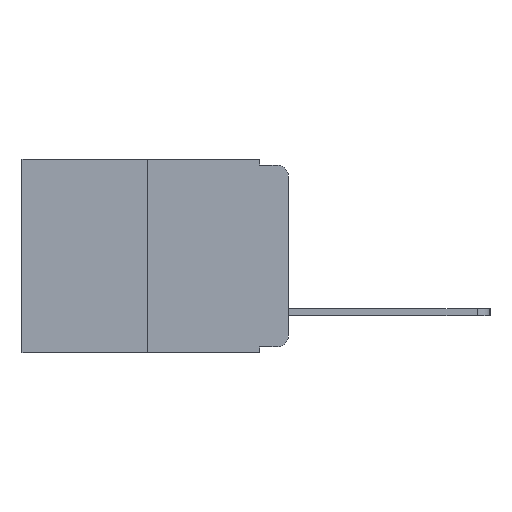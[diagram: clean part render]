
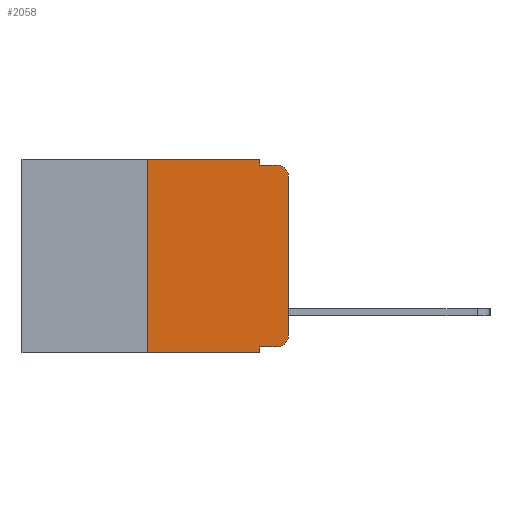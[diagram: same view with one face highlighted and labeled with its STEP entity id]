
A CAD part, left-side view. The second image highlights one B-rep face of the part: STEP entity #2058.
In plain terms, the highlighted planar face has unit normal (-1, 0, 0).
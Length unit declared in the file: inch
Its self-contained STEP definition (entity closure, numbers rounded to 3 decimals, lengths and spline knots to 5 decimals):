
#37 = CARTESIAN_POINT ( 'NONE',  ( 0., 0.473, 0. ) ) ;
#386 = VERTEX_POINT ( 'NONE', #9919 ) ;
#530 = CARTESIAN_POINT ( 'NONE',  ( 0., 0.051, -0.01 ) ) ;
#548 = CARTESIAN_POINT ( 'NONE',  ( 0., 0.25, -0.343 ) ) ;
#613 = CARTESIAN_POINT ( 'NONE',  ( 0., 0.25, 0. ) ) ;
#622 = CARTESIAN_POINT ( 'NONE',  ( 0., 0.051, -0.343 ) ) ;
#723 = VERTEX_POINT ( 'NONE', #8777 ) ;
#770 = EDGE_CURVE ( 'NONE', #386, #3956, #5890, .T. ) ;
#840 = CARTESIAN_POINT ( 'NONE',  ( 0., 0.051, 0. ) ) ;
#982 = AXIS2_PLACEMENT_3D ( 'NONE', #9594, #1736, #2177 ) ;
#1002 = EDGE_CURVE ( 'NONE', #3956, #3250, #6279, .T. ) ;
#1296 = VERTEX_POINT ( 'NONE', #622 ) ;
#1476 = VECTOR ( 'NONE', #10918, 39.37008 ) ;
#1736 = DIRECTION ( 'NONE',  ( -1., 0., 0. ) ) ;
#1944 = CARTESIAN_POINT ( 'NONE',  ( 0., 0.473, -0.343 ) ) ;
#2058 = ADVANCED_FACE ( 'NONE', ( #9789 ), #3217, .F. ) ;
#2126 = CARTESIAN_POINT ( 'NONE',  ( 0., 0.02, -0.03 ) ) ;
#2177 = DIRECTION ( 'NONE',  ( 0., 0., -1. ) ) ;
#2470 = DIRECTION ( 'NONE',  ( 0., 0., -1. ) ) ;
#2639 = CARTESIAN_POINT ( 'NONE',  ( 0., 0.051, 0. ) ) ;
#2712 = CIRCLE ( 'NONE', #9342, 0.02 ) ;
#2959 = DIRECTION ( 'NONE',  ( 0., -1., 0. ) ) ;
#3016 = ORIENTED_EDGE ( 'NONE', *, *, #10028, .T. ) ;
#3132 = DIRECTION ( 'NONE',  ( 0., 0., -1. ) ) ;
#3217 = PLANE ( 'NONE',  #4641 ) ;
#3250 = VERTEX_POINT ( 'NONE', #7295 ) ;
#3432 = VECTOR ( 'NONE', #5624, 39.37008 ) ;
#3616 = ORIENTED_EDGE ( 'NONE', *, *, #11093, .T. ) ;
#3637 = EDGE_CURVE ( 'NONE', #5778, #6204, #8328, .T. ) ;
#3664 = EDGE_CURVE ( 'NONE', #8264, #386, #10797, .T. ) ;
#3861 = VECTOR ( 'NONE', #7479, 39.37008 ) ;
#3956 = VERTEX_POINT ( 'NONE', #840 ) ;
#4050 = EDGE_LOOP ( 'NONE', ( #3016, #3616, #4286, #4614, #4967, #5254, #5357, #5860, #6402, #6733 ) ) ;
#4079 = LINE ( 'NONE', #2639, #1476 ) ;
#4286 = ORIENTED_EDGE ( 'NONE', *, *, #6363, .F. ) ;
#4368 = CARTESIAN_POINT ( 'NONE',  ( 0., 0.051, -0.333 ) ) ;
#4608 = CARTESIAN_POINT ( 'NONE',  ( 0., 0.02, -0.333 ) ) ;
#4614 = ORIENTED_EDGE ( 'NONE', *, *, #1002, .F. ) ;
#4641 = AXIS2_PLACEMENT_3D ( 'NONE', #37, #7239, #2470 ) ;
#4967 = ORIENTED_EDGE ( 'NONE', *, *, #770, .F. ) ;
#5078 = LINE ( 'NONE', #530, #9950 ) ;
#5254 = ORIENTED_EDGE ( 'NONE', *, *, #3664, .F. ) ;
#5357 = ORIENTED_EDGE ( 'NONE', *, *, #7666, .T. ) ;
#5373 = VECTOR ( 'NONE', #10734, 39.37008 ) ;
#5415 = EDGE_CURVE ( 'NONE', #9108, #1296, #4079, .T. ) ;
#5531 = DIRECTION ( 'NONE',  ( 0., -1., 0. ) ) ;
#5624 = DIRECTION ( 'NONE',  ( 0., -1., 0. ) ) ;
#5778 = VERTEX_POINT ( 'NONE', #4608 ) ;
#5860 = ORIENTED_EDGE ( 'NONE', *, *, #5415, .F. ) ;
#5890 = LINE ( 'NONE', #6013, #3432 ) ;
#6013 = CARTESIAN_POINT ( 'NONE',  ( 0., 0.473, 0. ) ) ;
#6204 = VERTEX_POINT ( 'NONE', #8804 ) ;
#6270 = VECTOR ( 'NONE', #6293, 39.37008 ) ;
#6279 = LINE ( 'NONE', #9103, #3861 ) ;
#6293 = DIRECTION ( 'NONE',  ( 0., 0., 1. ) ) ;
#6330 = CARTESIAN_POINT ( 'NONE',  ( 0., 0.02, -0.01 ) ) ;
#6363 = EDGE_CURVE ( 'NONE', #3250, #8302, #5078, .T. ) ;
#6402 = ORIENTED_EDGE ( 'NONE', *, *, #11432, .T. ) ;
#6509 = CARTESIAN_POINT ( 'NONE',  ( 0., 0., 0. ) ) ;
#6733 = ORIENTED_EDGE ( 'NONE', *, *, #3637, .T. ) ;
#7239 = DIRECTION ( 'NONE',  ( 1., 0., 0. ) ) ;
#7295 = CARTESIAN_POINT ( 'NONE',  ( 0., 0.051, -0.01 ) ) ;
#7479 = DIRECTION ( 'NONE',  ( 0., 0., -1. ) ) ;
#7666 = EDGE_CURVE ( 'NONE', #8264, #1296, #9923, .T. ) ;
#7689 = VECTOR ( 'NONE', #2959, 39.37008 ) ;
#8053 = DIRECTION ( 'NONE',  ( 0., -1., 0. ) ) ;
#8143 = CARTESIAN_POINT ( 'NONE',  ( 0., 0.051, -0.333 ) ) ;
#8264 = VERTEX_POINT ( 'NONE', #548 ) ;
#8302 = VERTEX_POINT ( 'NONE', #6330 ) ;
#8328 = CIRCLE ( 'NONE', #982, 0.02 ) ;
#8523 = DIRECTION ( 'NONE',  ( -1., 0., 0. ) ) ;
#8777 = CARTESIAN_POINT ( 'NONE',  ( 0., 0., -0.03 ) ) ;
#8804 = CARTESIAN_POINT ( 'NONE',  ( 0., 0., -0.313 ) ) ;
#9103 = CARTESIAN_POINT ( 'NONE',  ( 0., 0.051, 0. ) ) ;
#9108 = VERTEX_POINT ( 'NONE', #4368 ) ;
#9167 = VECTOR ( 'NONE', #5531, 39.37008 ) ;
#9342 = AXIS2_PLACEMENT_3D ( 'NONE', #2126, #8523, #3132 ) ;
#9594 = CARTESIAN_POINT ( 'NONE',  ( 0., 0.02, -0.313 ) ) ;
#9789 = FACE_OUTER_BOUND ( 'NONE', #4050, .T. ) ;
#9919 = CARTESIAN_POINT ( 'NONE',  ( 0., 0.25, 0. ) ) ;
#9923 = LINE ( 'NONE', #1944, #7689 ) ;
#9950 = VECTOR ( 'NONE', #8053, 39.37008 ) ;
#9965 = LINE ( 'NONE', #6509, #5373 ) ;
#10028 = EDGE_CURVE ( 'NONE', #6204, #723, #9965, .T. ) ;
#10319 = LINE ( 'NONE', #8143, #9167 ) ;
#10734 = DIRECTION ( 'NONE',  ( 0., 0., 1. ) ) ;
#10797 = LINE ( 'NONE', #613, #6270 ) ;
#10918 = DIRECTION ( 'NONE',  ( 0., 0., -1. ) ) ;
#11093 = EDGE_CURVE ( 'NONE', #723, #8302, #2712, .T. ) ;
#11432 = EDGE_CURVE ( 'NONE', #9108, #5778, #10319, .T. ) ;
